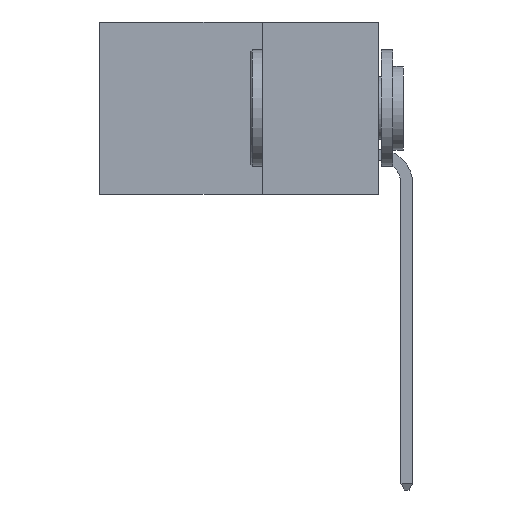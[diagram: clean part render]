
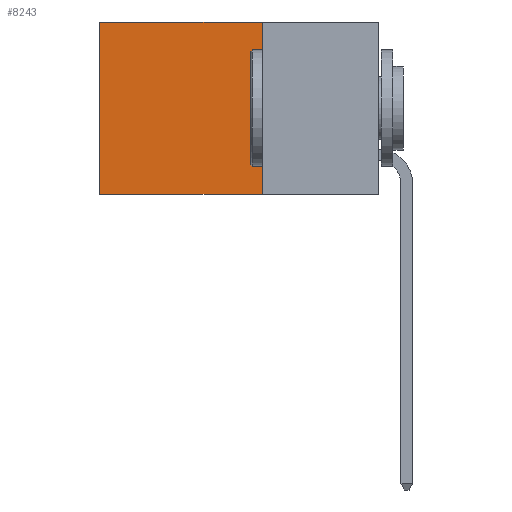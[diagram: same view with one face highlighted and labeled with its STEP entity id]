
A CAD part, left-side view. The second image highlights one B-rep face of the part: STEP entity #8243.
In plain terms, the highlighted planar face has unit normal (-1, 0, 0).
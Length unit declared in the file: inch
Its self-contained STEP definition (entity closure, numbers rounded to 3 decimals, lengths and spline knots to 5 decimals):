
#13 = CARTESIAN_POINT ( 'NONE',  ( 0.2615, 0.6, -0.37 ) ) ;
#804 = CARTESIAN_POINT ( 'NONE',  ( 0.2615, 0.6, 0. ) ) ;
#1369 = DIRECTION ( 'NONE',  ( 1., 0., 0. ) ) ;
#1489 = LINE ( 'NONE', #8574, #2312 ) ;
#2312 = VECTOR ( 'NONE', #9824, 39.37008 ) ;
#2533 = ORIENTED_EDGE ( 'NONE', *, *, #7005, .F. ) ;
#3310 = VECTOR ( 'NONE', #8003, 39.37008 ) ;
#4164 = CARTESIAN_POINT ( 'NONE',  ( 0.2615, 0.25, 0. ) ) ;
#4211 = ORIENTED_EDGE ( 'NONE', *, *, #13187, .T. ) ;
#5260 = VERTEX_POINT ( 'NONE', #13 ) ;
#5305 = CARTESIAN_POINT ( 'NONE',  ( 0.2615, 0.25, -0.37 ) ) ;
#5638 = FACE_OUTER_BOUND ( 'NONE', #11219, .T. ) ;
#5822 = ORIENTED_EDGE ( 'NONE', *, *, #12736, .T. ) ;
#6691 = CARTESIAN_POINT ( 'NONE',  ( 0.2615, 0.6, -0.37 ) ) ;
#6815 = CARTESIAN_POINT ( 'NONE',  ( 0.2615, 0.25, 0. ) ) ;
#7005 = EDGE_CURVE ( 'NONE', #7105, #7138, #15112, .T. ) ;
#7105 = VERTEX_POINT ( 'NONE', #4164 ) ;
#7138 = VERTEX_POINT ( 'NONE', #8182 ) ;
#7227 = LINE ( 'NONE', #6815, #10204 ) ;
#7914 = PLANE ( 'NONE',  #14773 ) ;
#8003 = DIRECTION ( 'NONE',  ( 0., 0., -1. ) ) ;
#8182 = CARTESIAN_POINT ( 'NONE',  ( 0.2615, 0.25, -0.37 ) ) ;
#8187 = DIRECTION ( 'NONE',  ( 0., 1., 0. ) ) ;
#8243 = ADVANCED_FACE ( 'NONE', ( #5638 ), #7914, .F. ) ;
#8574 = CARTESIAN_POINT ( 'NONE',  ( 0.2615, 0.25, -0.37 ) ) ;
#9187 = EDGE_CURVE ( 'NONE', #7138, #5260, #1489, .T. ) ;
#9216 = CARTESIAN_POINT ( 'NONE',  ( 0.2615, 0.25, -0.37 ) ) ;
#9618 = ORIENTED_EDGE ( 'NONE', *, *, #9187, .F. ) ;
#9824 = DIRECTION ( 'NONE',  ( 0., 1., 0. ) ) ;
#10192 = LINE ( 'NONE', #6691, #3310 ) ;
#10204 = VECTOR ( 'NONE', #8187, 39.37008 ) ;
#10454 = DIRECTION ( 'NONE',  ( 0., 0., -1. ) ) ;
#11219 = EDGE_LOOP ( 'NONE', ( #4211, #9618, #2533, #5822 ) ) ;
#11675 = VECTOR ( 'NONE', #11708, 39.37008 ) ;
#11708 = DIRECTION ( 'NONE',  ( 0., 0., -1. ) ) ;
#12736 = EDGE_CURVE ( 'NONE', #7105, #13566, #7227, .T. ) ;
#13187 = EDGE_CURVE ( 'NONE', #13566, #5260, #10192, .T. ) ;
#13566 = VERTEX_POINT ( 'NONE', #804 ) ;
#14773 = AXIS2_PLACEMENT_3D ( 'NONE', #9216, #1369, #10454 ) ;
#15112 = LINE ( 'NONE', #5305, #11675 ) ;
